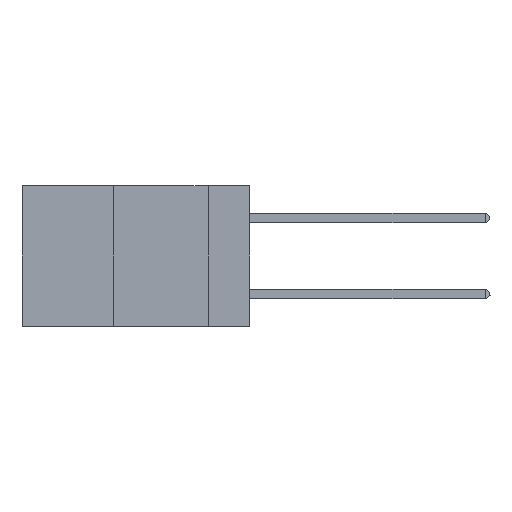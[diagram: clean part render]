
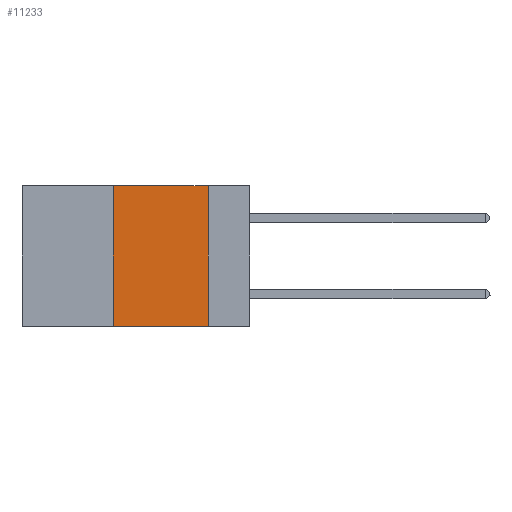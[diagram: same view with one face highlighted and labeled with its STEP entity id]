
A CAD part, left-side view. The second image highlights one B-rep face of the part: STEP entity #11233.
In plain terms, the highlighted planar face has unit normal (-1, 0, 0).
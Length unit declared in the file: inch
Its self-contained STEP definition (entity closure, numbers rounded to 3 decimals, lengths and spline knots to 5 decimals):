
#510 = LINE ( 'NONE', #13742, #9636 ) ;
#668 = EDGE_CURVE ( 'NONE', #880, #8923, #510, .T. ) ;
#880 = VERTEX_POINT ( 'NONE', #3210 ) ;
#1494 = CARTESIAN_POINT ( 'NONE',  ( 0., 0.11, -0.37 ) ) ;
#1548 = ORIENTED_EDGE ( 'NONE', *, *, #7561, .T. ) ;
#1692 = CARTESIAN_POINT ( 'NONE',  ( 0., 0.6, -0.37 ) ) ;
#2995 = LINE ( 'NONE', #9557, #5222 ) ;
#3045 = LINE ( 'NONE', #1692, #10142 ) ;
#3210 = CARTESIAN_POINT ( 'NONE',  ( 0., 0.36, -0.37 ) ) ;
#3866 = ORIENTED_EDGE ( 'NONE', *, *, #9012, .F. ) ;
#4039 = CARTESIAN_POINT ( 'NONE',  ( 0., 0.36, 0. ) ) ;
#4546 = EDGE_CURVE ( 'NONE', #8923, #5404, #12367, .T. ) ;
#5222 = VECTOR ( 'NONE', #14837, 39.37008 ) ;
#5404 = VERTEX_POINT ( 'NONE', #12286 ) ;
#5458 = VECTOR ( 'NONE', #10588, 39.37008 ) ;
#5954 = DIRECTION ( 'NONE',  ( 1., 0., 0. ) ) ;
#6382 = AXIS2_PLACEMENT_3D ( 'NONE', #9929, #5954, #9875 ) ;
#6674 = CARTESIAN_POINT ( 'NONE',  ( 0., 0.6, 0. ) ) ;
#6891 = VERTEX_POINT ( 'NONE', #1494 ) ;
#7101 = DIRECTION ( 'NONE',  ( 0., 0., 1. ) ) ;
#7561 = EDGE_CURVE ( 'NONE', #880, #6891, #3045, .T. ) ;
#8923 = VERTEX_POINT ( 'NONE', #4039 ) ;
#9012 = EDGE_CURVE ( 'NONE', #5404, #6891, #2995, .T. ) ;
#9557 = CARTESIAN_POINT ( 'NONE',  ( 0., 0.11, 0. ) ) ;
#9636 = VECTOR ( 'NONE', #7101, 39.37008 ) ;
#9875 = DIRECTION ( 'NONE',  ( 0., 0., -1. ) ) ;
#9929 = CARTESIAN_POINT ( 'NONE',  ( 0., 0.6, 0. ) ) ;
#10142 = VECTOR ( 'NONE', #13433, 39.37008 ) ;
#10241 = FACE_OUTER_BOUND ( 'NONE', #10342, .T. ) ;
#10342 = EDGE_LOOP ( 'NONE', ( #3866, #10377, #15816, #1548 ) ) ;
#10377 = ORIENTED_EDGE ( 'NONE', *, *, #4546, .F. ) ;
#10588 = DIRECTION ( 'NONE',  ( 0., -1., 0. ) ) ;
#11233 = ADVANCED_FACE ( 'NONE', ( #10241 ), #12473, .F. ) ;
#12286 = CARTESIAN_POINT ( 'NONE',  ( 0., 0.11, 0. ) ) ;
#12367 = LINE ( 'NONE', #6674, #5458 ) ;
#12473 = PLANE ( 'NONE',  #6382 ) ;
#13433 = DIRECTION ( 'NONE',  ( 0., -1., 0. ) ) ;
#13742 = CARTESIAN_POINT ( 'NONE',  ( 0., 0.36, 0. ) ) ;
#14837 = DIRECTION ( 'NONE',  ( 0., 0., -1. ) ) ;
#15816 = ORIENTED_EDGE ( 'NONE', *, *, #668, .F. ) ;
